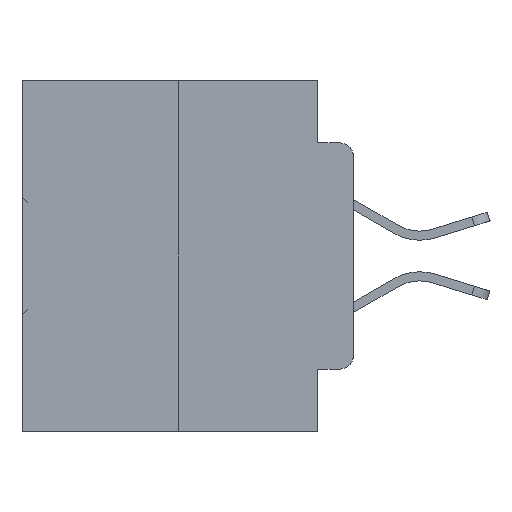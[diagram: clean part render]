
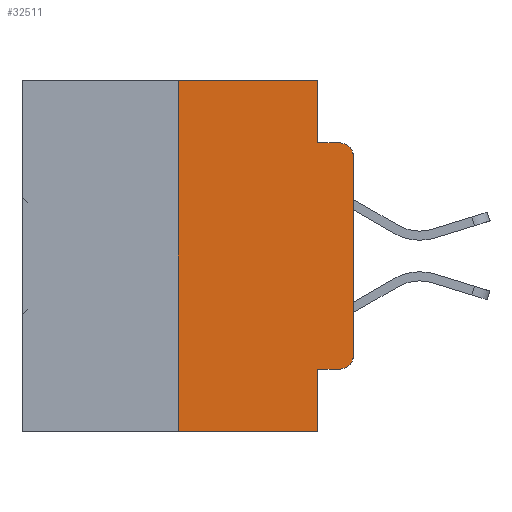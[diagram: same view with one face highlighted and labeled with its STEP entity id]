
A CAD part, left-side view. The second image highlights one B-rep face of the part: STEP entity #32511.
In plain terms, the highlighted planar face has unit normal (-1, 0, 0).
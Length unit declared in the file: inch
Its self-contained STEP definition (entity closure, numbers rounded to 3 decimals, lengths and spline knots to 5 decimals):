
#113 = EDGE_CURVE ( 'NONE', #12592, #20767, #16880, .T. ) ;
#187 = ORIENTED_EDGE ( 'NONE', *, *, #35105, .F. ) ;
#565 = LINE ( 'NONE', #15557, #15154 ) ;
#610 = CARTESIAN_POINT ( 'NONE',  ( 0., 0.473, 0. ) ) ;
#626 = CARTESIAN_POINT ( 'NONE',  ( 0., 0.051, -0.5 ) ) ;
#666 = EDGE_CURVE ( 'NONE', #14118, #4514, #565, .T. ) ;
#929 = DIRECTION ( 'NONE',  ( 0., 0., 1. ) ) ;
#1254 = LINE ( 'NONE', #31714, #15820 ) ;
#2340 = ORIENTED_EDGE ( 'NONE', *, *, #18946, .F. ) ;
#3677 = AXIS2_PLACEMENT_3D ( 'NONE', #21605, #5315, #24317 ) ;
#4315 = CARTESIAN_POINT ( 'NONE',  ( 0., 0.473, -0.5 ) ) ;
#4514 = VERTEX_POINT ( 'NONE', #17401 ) ;
#4867 = LINE ( 'NONE', #20080, #17653 ) ;
#4942 = ORIENTED_EDGE ( 'NONE', *, *, #666, .T. ) ;
#5315 = DIRECTION ( 'NONE',  ( -1., 0., 0. ) ) ;
#6828 = DIRECTION ( 'NONE',  ( 0., -1., 0. ) ) ;
#7630 = CARTESIAN_POINT ( 'NONE',  ( 0., 0.02, -0.3915 ) ) ;
#7899 = CIRCLE ( 'NONE', #3677, 0.02 ) ;
#8082 = CARTESIAN_POINT ( 'NONE',  ( 0., 0., -0.3915 ) ) ;
#8483 = LINE ( 'NONE', #34639, #29289 ) ;
#8891 = DIRECTION ( 'NONE',  ( 0., 0., -1. ) ) ;
#8906 = CARTESIAN_POINT ( 'NONE',  ( 0., 0.051, -0.0885 ) ) ;
#9770 = DIRECTION ( 'NONE',  ( 0., -1., 0. ) ) ;
#9781 = CARTESIAN_POINT ( 'NONE',  ( 0., 0.051, 0. ) ) ;
#9894 = DIRECTION ( 'NONE',  ( 0., 0., -1. ) ) ;
#9980 = VERTEX_POINT ( 'NONE', #12598 ) ;
#10347 = DIRECTION ( 'NONE',  ( 0., 0., -1. ) ) ;
#11413 = LINE ( 'NONE', #31247, #32143 ) ;
#12175 = CARTESIAN_POINT ( 'NONE',  ( 0., 0.25, -0.5 ) ) ;
#12592 = VERTEX_POINT ( 'NONE', #17677 ) ;
#12598 = CARTESIAN_POINT ( 'NONE',  ( 0., 0.02, -0.4115 ) ) ;
#13030 = ORIENTED_EDGE ( 'NONE', *, *, #32904, .T. ) ;
#13199 = LINE ( 'NONE', #4315, #26773 ) ;
#13891 = CARTESIAN_POINT ( 'NONE',  ( 0., 0.051, -0.4115 ) ) ;
#14118 = VERTEX_POINT ( 'NONE', #8082 ) ;
#14155 = PLANE ( 'NONE',  #25081 ) ;
#15154 = VECTOR ( 'NONE', #15417, 39.37008 ) ;
#15197 = FACE_OUTER_BOUND ( 'NONE', #20240, .T. ) ;
#15417 = DIRECTION ( 'NONE',  ( 0., 0., 1. ) ) ;
#15557 = CARTESIAN_POINT ( 'NONE',  ( 0., 0., 0. ) ) ;
#15820 = VECTOR ( 'NONE', #16005, 39.37008 ) ;
#16005 = DIRECTION ( 'NONE',  ( 0., -1., 0. ) ) ;
#16620 = DIRECTION ( 'NONE',  ( 0., -1., 0. ) ) ;
#16880 = LINE ( 'NONE', #9781, #24082 ) ;
#17314 = ORIENTED_EDGE ( 'NONE', *, *, #113, .F. ) ;
#17401 = CARTESIAN_POINT ( 'NONE',  ( 0., 0., -0.1085 ) ) ;
#17653 = VECTOR ( 'NONE', #929, 39.37008 ) ;
#17677 = CARTESIAN_POINT ( 'NONE',  ( 0., 0.051, 0. ) ) ;
#18064 = VERTEX_POINT ( 'NONE', #28238 ) ;
#18225 = ORIENTED_EDGE ( 'NONE', *, *, #30408, .T. ) ;
#18946 = EDGE_CURVE ( 'NONE', #28502, #12592, #1254, .T. ) ;
#19401 = EDGE_CURVE ( 'NONE', #20158, #20736, #13199, .T. ) ;
#19481 = ORIENTED_EDGE ( 'NONE', *, *, #23660, .F. ) ;
#20080 = CARTESIAN_POINT ( 'NONE',  ( 0., 0.25, 0. ) ) ;
#20158 = VERTEX_POINT ( 'NONE', #12175 ) ;
#20240 = EDGE_LOOP ( 'NONE', ( #4942, #13030, #34567, #17314, #2340, #19481, #21163, #187, #18225, #34219 ) ) ;
#20736 = VERTEX_POINT ( 'NONE', #626 ) ;
#20767 = VERTEX_POINT ( 'NONE', #8906 ) ;
#21144 = DIRECTION ( 'NONE',  ( 0., 0., -1. ) ) ;
#21163 = ORIENTED_EDGE ( 'NONE', *, *, #19401, .T. ) ;
#21605 = CARTESIAN_POINT ( 'NONE',  ( 0., 0.02, -0.1085 ) ) ;
#23660 = EDGE_CURVE ( 'NONE', #20158, #28502, #4867, .T. ) ;
#24082 = VECTOR ( 'NONE', #9894, 39.37008 ) ;
#24317 = DIRECTION ( 'NONE',  ( 0., 0., -1. ) ) ;
#25081 = AXIS2_PLACEMENT_3D ( 'NONE', #610, #25180, #8891 ) ;
#25175 = CARTESIAN_POINT ( 'NONE',  ( 0., 0.02, -0.0885 ) ) ;
#25180 = DIRECTION ( 'NONE',  ( 1., 0., 0. ) ) ;
#25515 = VECTOR ( 'NONE', #16620, 39.37008 ) ;
#26074 = CIRCLE ( 'NONE', #34835, 0.02 ) ;
#26206 = VERTEX_POINT ( 'NONE', #25175 ) ;
#26605 = DIRECTION ( 'NONE',  ( -1., 0., 0. ) ) ;
#26773 = VECTOR ( 'NONE', #9770, 39.37008 ) ;
#27047 = EDGE_CURVE ( 'NONE', #20767, #26206, #11413, .T. ) ;
#27725 = EDGE_CURVE ( 'NONE', #9980, #14118, #26074, .T. ) ;
#28238 = CARTESIAN_POINT ( 'NONE',  ( 0., 0.051, -0.4115 ) ) ;
#28502 = VERTEX_POINT ( 'NONE', #32302 ) ;
#29289 = VECTOR ( 'NONE', #21144, 39.37008 ) ;
#30408 = EDGE_CURVE ( 'NONE', #18064, #9980, #33508, .T. ) ;
#31247 = CARTESIAN_POINT ( 'NONE',  ( 0., 0.051, -0.0885 ) ) ;
#31714 = CARTESIAN_POINT ( 'NONE',  ( 0., 0.473, 0. ) ) ;
#32143 = VECTOR ( 'NONE', #6828, 39.37008 ) ;
#32302 = CARTESIAN_POINT ( 'NONE',  ( 0., 0.25, 0. ) ) ;
#32511 = ADVANCED_FACE ( 'NONE', ( #15197 ), #14155, .F. ) ;
#32904 = EDGE_CURVE ( 'NONE', #4514, #26206, #7899, .T. ) ;
#33508 = LINE ( 'NONE', #13891, #25515 ) ;
#34219 = ORIENTED_EDGE ( 'NONE', *, *, #27725, .T. ) ;
#34567 = ORIENTED_EDGE ( 'NONE', *, *, #27047, .F. ) ;
#34639 = CARTESIAN_POINT ( 'NONE',  ( 0., 0.051, 0. ) ) ;
#34835 = AXIS2_PLACEMENT_3D ( 'NONE', #7630, #26605, #10347 ) ;
#35105 = EDGE_CURVE ( 'NONE', #18064, #20736, #8483, .T. ) ;
